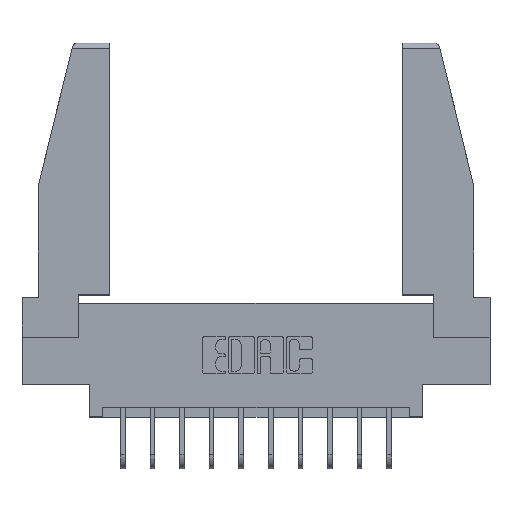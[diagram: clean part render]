
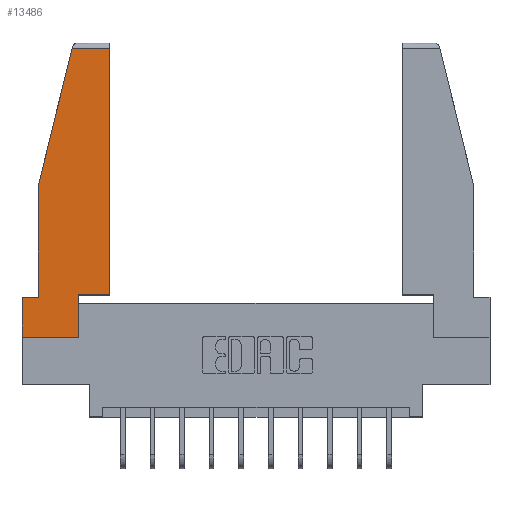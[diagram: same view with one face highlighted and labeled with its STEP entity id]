
A CAD part, top view. The second image highlights one B-rep face of the part: STEP entity #13486.
In plain terms, the highlighted planar face has unit normal (0, 0, 1).
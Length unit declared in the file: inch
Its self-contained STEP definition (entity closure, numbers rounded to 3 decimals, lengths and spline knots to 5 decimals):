
#466 = EDGE_CURVE ( 'NONE', #4517, #4797, #6647, .T. ) ;
#638 = LINE ( 'NONE', #10678, #8372 ) ;
#644 = DIRECTION ( 'NONE',  ( 0., 0., 1. ) ) ;
#782 = CARTESIAN_POINT ( 'NONE',  ( 0.2636, 1.52, 0. ) ) ;
#1219 = CARTESIAN_POINT ( 'NONE',  ( 0.297, 0.223, 0. ) ) ;
#1298 = ORIENTED_EDGE ( 'NONE', *, *, #12942, .T. ) ;
#1824 = LINE ( 'NONE', #1219, #12856 ) ;
#1895 = CARTESIAN_POINT ( 'NONE',  ( 0.297, 0., 0. ) ) ;
#1920 = VECTOR ( 'NONE', #8090, 39.37008 ) ;
#2075 = EDGE_LOOP ( 'NONE', ( #11309, #12546, #6874, #6093, #1298, #12654, #13816, #2180, #8234 ) ) ;
#2180 = ORIENTED_EDGE ( 'NONE', *, *, #466, .T. ) ;
#2250 = LINE ( 'NONE', #6440, #2598 ) ;
#2439 = CARTESIAN_POINT ( 'NONE',  ( 0.461, 1.52, 0. ) ) ;
#2598 = VECTOR ( 'NONE', #5374, 39.37008 ) ;
#2612 = CARTESIAN_POINT ( 'NONE',  ( 0., 0.21, 0. ) ) ;
#2642 = VERTEX_POINT ( 'NONE', #782 ) ;
#2657 = PLANE ( 'NONE',  #14131 ) ;
#3189 = VERTEX_POINT ( 'NONE', #8799 ) ;
#3457 = VECTOR ( 'NONE', #9289, 39.37008 ) ;
#3608 = VECTOR ( 'NONE', #12355, 39.37008 ) ;
#3732 = VECTOR ( 'NONE', #7261, 39.37008 ) ;
#4232 = LINE ( 'NONE', #5414, #4922 ) ;
#4517 = VERTEX_POINT ( 'NONE', #1895 ) ;
#4634 = DIRECTION ( 'NONE',  ( 0., -1., 0. ) ) ;
#4700 = LINE ( 'NONE', #10297, #10417 ) ;
#4797 = VERTEX_POINT ( 'NONE', #9199 ) ;
#4922 = VECTOR ( 'NONE', #6429, 39.37008 ) ;
#5119 = EDGE_CURVE ( 'NONE', #10136, #4517, #638, .T. ) ;
#5300 = LINE ( 'NONE', #10503, #1920 ) ;
#5374 = DIRECTION ( 'NONE',  ( 0., 1., 0. ) ) ;
#5414 = CARTESIAN_POINT ( 'NONE',  ( 0., 1.52, 0. ) ) ;
#5538 = EDGE_CURVE ( 'NONE', #2642, #7988, #5300, .T. ) ;
#5641 = FACE_OUTER_BOUND ( 'NONE', #2075, .T. ) ;
#6074 = DIRECTION ( 'NONE',  ( 1., 0., 0. ) ) ;
#6093 = ORIENTED_EDGE ( 'NONE', *, *, #10839, .T. ) ;
#6429 = DIRECTION ( 'NONE',  ( -1., 0., 0. ) ) ;
#6440 = CARTESIAN_POINT ( 'NONE',  ( 0.461, 0.223, 0. ) ) ;
#6497 = LINE ( 'NONE', #6998, #3608 ) ;
#6647 = LINE ( 'NONE', #7070, #3732 ) ;
#6874 = ORIENTED_EDGE ( 'NONE', *, *, #5538, .T. ) ;
#6998 = CARTESIAN_POINT ( 'NONE',  ( 0.086, 0.8, 0. ) ) ;
#7070 = CARTESIAN_POINT ( 'NONE',  ( 0.297, 0., 0. ) ) ;
#7187 = CARTESIAN_POINT ( 'NONE',  ( 0., 0., 0. ) ) ;
#7192 = LINE ( 'NONE', #2612, #3457 ) ;
#7219 = EDGE_CURVE ( 'NONE', #4797, #3189, #1824, .T. ) ;
#7261 = DIRECTION ( 'NONE',  ( 0., 1., 0. ) ) ;
#7988 = VERTEX_POINT ( 'NONE', #11707 ) ;
#8090 = DIRECTION ( 'NONE',  ( -0.239, -0.971, 0. ) ) ;
#8234 = ORIENTED_EDGE ( 'NONE', *, *, #7219, .T. ) ;
#8372 = VECTOR ( 'NONE', #9671, 39.37008 ) ;
#8622 = EDGE_CURVE ( 'NONE', #14007, #10136, #4700, .T. ) ;
#8799 = CARTESIAN_POINT ( 'NONE',  ( 0.461, 0.223, 0. ) ) ;
#8808 = DIRECTION ( 'NONE',  ( 1., 0., 0. ) ) ;
#9199 = CARTESIAN_POINT ( 'NONE',  ( 0.297, 0.223, 0. ) ) ;
#9289 = DIRECTION ( 'NONE',  ( -1., 0., 0. ) ) ;
#9389 = CARTESIAN_POINT ( 'NONE',  ( 0., 0.21, 0. ) ) ;
#9671 = DIRECTION ( 'NONE',  ( 1., 0., 0. ) ) ;
#10136 = VERTEX_POINT ( 'NONE', #11257 ) ;
#10297 = CARTESIAN_POINT ( 'NONE',  ( 0., 0.21, 0. ) ) ;
#10368 = VERTEX_POINT ( 'NONE', #2439 ) ;
#10417 = VECTOR ( 'NONE', #4634, 39.37008 ) ;
#10503 = CARTESIAN_POINT ( 'NONE',  ( 0.271, 1.55, 0. ) ) ;
#10678 = CARTESIAN_POINT ( 'NONE',  ( 0., 0., 0. ) ) ;
#10839 = EDGE_CURVE ( 'NONE', #7988, #11358, #6497, .T. ) ;
#11257 = CARTESIAN_POINT ( 'NONE',  ( 0., 0., 0. ) ) ;
#11309 = ORIENTED_EDGE ( 'NONE', *, *, #13039, .T. ) ;
#11358 = VERTEX_POINT ( 'NONE', #11778 ) ;
#11707 = CARTESIAN_POINT ( 'NONE',  ( 0.086, 0.8, 0. ) ) ;
#11778 = CARTESIAN_POINT ( 'NONE',  ( 0.086, 0.21, 0. ) ) ;
#12355 = DIRECTION ( 'NONE',  ( 0., -1., 0. ) ) ;
#12546 = ORIENTED_EDGE ( 'NONE', *, *, #14256, .T. ) ;
#12654 = ORIENTED_EDGE ( 'NONE', *, *, #8622, .T. ) ;
#12856 = VECTOR ( 'NONE', #8808, 39.37008 ) ;
#12942 = EDGE_CURVE ( 'NONE', #11358, #14007, #7192, .T. ) ;
#13039 = EDGE_CURVE ( 'NONE', #3189, #10368, #2250, .T. ) ;
#13486 = ADVANCED_FACE ( 'NONE', ( #5641 ), #2657, .T. ) ;
#13816 = ORIENTED_EDGE ( 'NONE', *, *, #5119, .T. ) ;
#14007 = VERTEX_POINT ( 'NONE', #9389 ) ;
#14131 = AXIS2_PLACEMENT_3D ( 'NONE', #7187, #644, #6074 ) ;
#14256 = EDGE_CURVE ( 'NONE', #10368, #2642, #4232, .T. ) ;
